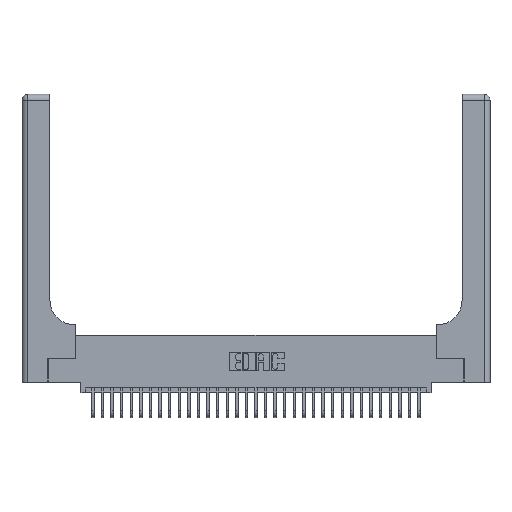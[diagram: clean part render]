
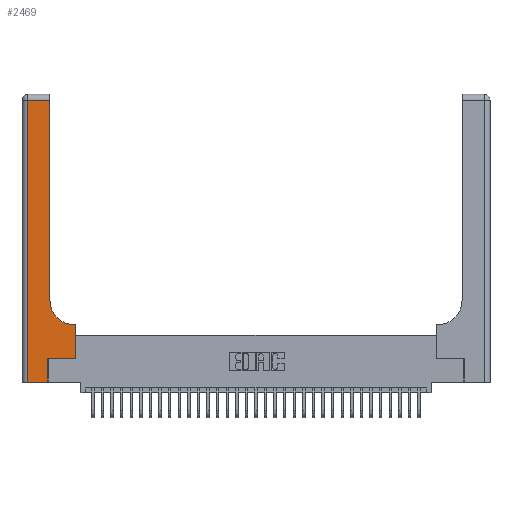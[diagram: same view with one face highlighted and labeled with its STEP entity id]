
A CAD part, top view. The second image highlights one B-rep face of the part: STEP entity #2469.
In plain terms, the highlighted planar face has unit normal (0, 0, 1).
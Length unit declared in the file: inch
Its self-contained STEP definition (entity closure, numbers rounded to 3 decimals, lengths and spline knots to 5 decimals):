
#70 = CARTESIAN_POINT ( 'NONE',  ( 0.2915, 0.85, 0.37 ) ) ;
#331 = CARTESIAN_POINT ( 'NONE',  ( 0., 2.94, 0.37 ) ) ;
#1157 = EDGE_CURVE ( 'NONE', #26710, #31792, #28815, .T. ) ;
#1273 = ORIENTED_EDGE ( 'NONE', *, *, #11327, .T. ) ;
#1412 = DIRECTION ( 'NONE',  ( 0., -1., 0. ) ) ;
#1556 = EDGE_CURVE ( 'NONE', #31792, #29283, #24465, .T. ) ;
#1647 = DIRECTION ( 'NONE',  ( 0., 0., -1. ) ) ;
#2469 = ADVANCED_FACE ( 'NONE', ( #8583 ), #16814, .F. ) ;
#2870 = VERTEX_POINT ( 'NONE', #13243 ) ;
#2977 = DIRECTION ( 'NONE',  ( 1., 0., 0. ) ) ;
#3033 = EDGE_CURVE ( 'NONE', #26142, #26710, #32216, .T. ) ;
#3331 = VECTOR ( 'NONE', #5383, 39.37008 ) ;
#3824 = CARTESIAN_POINT ( 'NONE',  ( 0.5415, 0.85, 0.37 ) ) ;
#4288 = VECTOR ( 'NONE', #11887, 39.37008 ) ;
#4910 = LINE ( 'NONE', #331, #3331 ) ;
#5074 = CARTESIAN_POINT ( 'NONE',  ( 0.06, 2.94, 0.37 ) ) ;
#5383 = DIRECTION ( 'NONE',  ( -1., 0., 0. ) ) ;
#5650 = ORIENTED_EDGE ( 'NONE', *, *, #1157, .T. ) ;
#5750 = VERTEX_POINT ( 'NONE', #21027 ) ;
#6296 = CARTESIAN_POINT ( 'NONE',  ( 0.269, 0., 0.37 ) ) ;
#6362 = DIRECTION ( 'NONE',  ( 1., 0., 0. ) ) ;
#6505 = CARTESIAN_POINT ( 'NONE',  ( 0., 3., 0.37 ) ) ;
#7240 = CARTESIAN_POINT ( 'NONE',  ( 0.269, 0., 0.37 ) ) ;
#7318 = DIRECTION ( 'NONE',  ( 1., 0., 0. ) ) ;
#7518 = AXIS2_PLACEMENT_3D ( 'NONE', #3824, #21536, #6362 ) ;
#7662 = ORIENTED_EDGE ( 'NONE', *, *, #3033, .T. ) ;
#8583 = FACE_OUTER_BOUND ( 'NONE', #25543, .T. ) ;
#8651 = DIRECTION ( 'NONE',  ( 0., 1., 0. ) ) ;
#10610 = ORIENTED_EDGE ( 'NONE', *, *, #32601, .T. ) ;
#10630 = VERTEX_POINT ( 'NONE', #11605 ) ;
#10958 = AXIS2_PLACEMENT_3D ( 'NONE', #6505, #1647, #19348 ) ;
#11327 = EDGE_CURVE ( 'NONE', #10630, #19420, #31147, .T. ) ;
#11605 = CARTESIAN_POINT ( 'NONE',  ( 0.5585, 0.6, 0.37 ) ) ;
#11887 = DIRECTION ( 'NONE',  ( -1., 0., 0. ) ) ;
#12909 = VECTOR ( 'NONE', #1412, 39.37008 ) ;
#13243 = CARTESIAN_POINT ( 'NONE',  ( 0.5585, 0.25, 0.37 ) ) ;
#14014 = CARTESIAN_POINT ( 'NONE',  ( 0.06, 3., 0.37 ) ) ;
#14132 = EDGE_CURVE ( 'NONE', #19420, #16333, #26293, .T. ) ;
#14675 = EDGE_CURVE ( 'NONE', #2870, #10630, #29014, .T. ) ;
#15414 = VECTOR ( 'NONE', #7318, 39.37008 ) ;
#15531 = ORIENTED_EDGE ( 'NONE', *, *, #29630, .T. ) ;
#15894 = CARTESIAN_POINT ( 'NONE',  ( 0.2915, 3., 0.37 ) ) ;
#16333 = VERTEX_POINT ( 'NONE', #70 ) ;
#16814 = PLANE ( 'NONE',  #10958 ) ;
#16968 = VECTOR ( 'NONE', #29041, 39.37008 ) ;
#17600 = LINE ( 'NONE', #18157, #31775 ) ;
#18157 = CARTESIAN_POINT ( 'NONE',  ( 0.269, 0.25, 0.37 ) ) ;
#18511 = CARTESIAN_POINT ( 'NONE',  ( 0.5415, 0.6, 0.37 ) ) ;
#19142 = ORIENTED_EDGE ( 'NONE', *, *, #1556, .T. ) ;
#19244 = CARTESIAN_POINT ( 'NONE',  ( 0.269, 0.25, 0.37 ) ) ;
#19348 = DIRECTION ( 'NONE',  ( -1., 0., 0. ) ) ;
#19395 = CARTESIAN_POINT ( 'NONE',  ( 0.2915, 0.6, 0.37 ) ) ;
#19420 = VERTEX_POINT ( 'NONE', #18511 ) ;
#19639 = ORIENTED_EDGE ( 'NONE', *, *, #14132, .T. ) ;
#20045 = CARTESIAN_POINT ( 'NONE',  ( 0., 0., 0.37 ) ) ;
#20558 = ORIENTED_EDGE ( 'NONE', *, *, #14675, .T. ) ;
#20682 = EDGE_CURVE ( 'NONE', #16333, #5750, #29103, .T. ) ;
#21027 = CARTESIAN_POINT ( 'NONE',  ( 0.2915, 2.94, 0.37 ) ) ;
#21278 = CARTESIAN_POINT ( 'NONE',  ( 0.5585, 0.25, 0.37 ) ) ;
#21536 = DIRECTION ( 'NONE',  ( 0., 0., -1. ) ) ;
#21546 = VECTOR ( 'NONE', #8651, 39.37008 ) ;
#22414 = VECTOR ( 'NONE', #23515, 39.37008 ) ;
#23515 = DIRECTION ( 'NONE',  ( 0., 1., 0. ) ) ;
#24465 = LINE ( 'NONE', #6296, #16968 ) ;
#25543 = EDGE_LOOP ( 'NONE', ( #27950, #15531, #7662, #5650, #19142, #10610, #20558, #1273, #19639 ) ) ;
#26142 = VERTEX_POINT ( 'NONE', #5074 ) ;
#26293 = CIRCLE ( 'NONE', #7518, 0.25 ) ;
#26710 = VERTEX_POINT ( 'NONE', #30094 ) ;
#27950 = ORIENTED_EDGE ( 'NONE', *, *, #20682, .T. ) ;
#28815 = LINE ( 'NONE', #20045, #15414 ) ;
#29014 = LINE ( 'NONE', #21278, #21546 ) ;
#29041 = DIRECTION ( 'NONE',  ( 0., 1., 0. ) ) ;
#29103 = LINE ( 'NONE', #15894, #22414 ) ;
#29283 = VERTEX_POINT ( 'NONE', #19244 ) ;
#29630 = EDGE_CURVE ( 'NONE', #5750, #26142, #4910, .T. ) ;
#30094 = CARTESIAN_POINT ( 'NONE',  ( 0.06, 0., 0.37 ) ) ;
#31147 = LINE ( 'NONE', #19395, #4288 ) ;
#31775 = VECTOR ( 'NONE', #2977, 39.37008 ) ;
#31792 = VERTEX_POINT ( 'NONE', #7240 ) ;
#32216 = LINE ( 'NONE', #14014, #12909 ) ;
#32601 = EDGE_CURVE ( 'NONE', #29283, #2870, #17600, .T. ) ;
